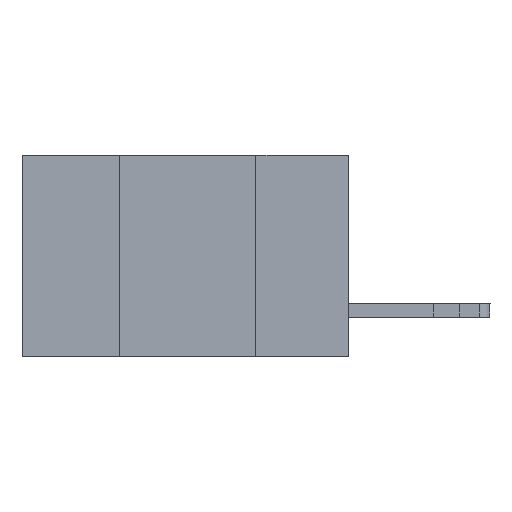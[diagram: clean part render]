
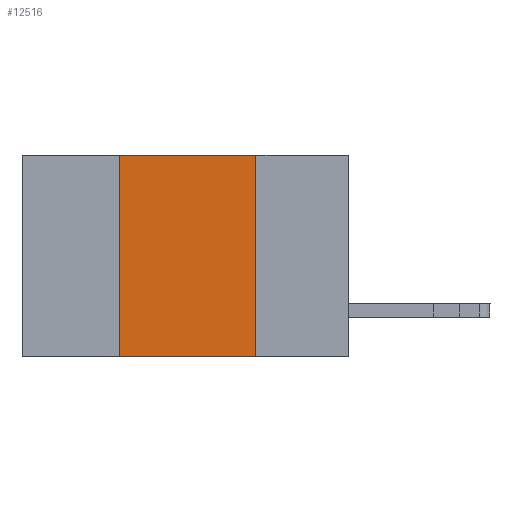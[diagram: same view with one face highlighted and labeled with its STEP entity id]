
A CAD part, left-side view. The second image highlights one B-rep face of the part: STEP entity #12516.
In plain terms, the highlighted planar face has unit normal (-1, 0, 0).
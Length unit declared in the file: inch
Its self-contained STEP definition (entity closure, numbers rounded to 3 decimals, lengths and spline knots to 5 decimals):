
#341 = DIRECTION ( 'NONE',  ( 1., 0., 0. ) ) ;
#452 = CARTESIAN_POINT ( 'NONE',  ( 0., 0.6, 0. ) ) ;
#562 = DIRECTION ( 'NONE',  ( 0., 0., -1. ) ) ;
#1855 = DIRECTION ( 'NONE',  ( 0., 0., 1. ) ) ;
#4172 = VERTEX_POINT ( 'NONE', #7722 ) ;
#4408 = CARTESIAN_POINT ( 'NONE',  ( 0., 0.17, 0. ) ) ;
#4978 = PLANE ( 'NONE',  #6193 ) ;
#5521 = VECTOR ( 'NONE', #16420, 39.37008 ) ;
#5576 = CARTESIAN_POINT ( 'NONE',  ( 0., 0.17, 0. ) ) ;
#6193 = AXIS2_PLACEMENT_3D ( 'NONE', #452, #341, #562 ) ;
#6231 = EDGE_CURVE ( 'NONE', #17138, #4172, #17937, .T. ) ;
#7722 = CARTESIAN_POINT ( 'NONE',  ( 0., 0.42, 0. ) ) ;
#9552 = VECTOR ( 'NONE', #20217, 39.37008 ) ;
#9695 = EDGE_CURVE ( 'NONE', #17138, #19315, #11885, .T. ) ;
#9829 = ORIENTED_EDGE ( 'NONE', *, *, #19598, .F. ) ;
#9984 = LINE ( 'NONE', #11988, #5521 ) ;
#10216 = FACE_OUTER_BOUND ( 'NONE', #20746, .T. ) ;
#11525 = CARTESIAN_POINT ( 'NONE',  ( 0., 0.42, -0.37 ) ) ;
#11875 = VERTEX_POINT ( 'NONE', #4408 ) ;
#11885 = LINE ( 'NONE', #20127, #12164 ) ;
#11988 = CARTESIAN_POINT ( 'NONE',  ( 0., 0.6, 0. ) ) ;
#12164 = VECTOR ( 'NONE', #18324, 39.37008 ) ;
#12516 = ADVANCED_FACE ( 'NONE', ( #10216 ), #4978, .F. ) ;
#12523 = CARTESIAN_POINT ( 'NONE',  ( 0., 0.17, -0.37 ) ) ;
#13143 = EDGE_CURVE ( 'NONE', #11875, #19315, #13459, .T. ) ;
#13459 = LINE ( 'NONE', #5576, #9552 ) ;
#13522 = ORIENTED_EDGE ( 'NONE', *, *, #13143, .F. ) ;
#15099 = ORIENTED_EDGE ( 'NONE', *, *, #9695, .T. ) ;
#15252 = VECTOR ( 'NONE', #1855, 39.37008 ) ;
#15391 = ORIENTED_EDGE ( 'NONE', *, *, #6231, .F. ) ;
#16256 = CARTESIAN_POINT ( 'NONE',  ( 0., 0.42, 0. ) ) ;
#16420 = DIRECTION ( 'NONE',  ( 0., -1., 0. ) ) ;
#17138 = VERTEX_POINT ( 'NONE', #11525 ) ;
#17937 = LINE ( 'NONE', #16256, #15252 ) ;
#18324 = DIRECTION ( 'NONE',  ( 0., -1., 0. ) ) ;
#19315 = VERTEX_POINT ( 'NONE', #12523 ) ;
#19598 = EDGE_CURVE ( 'NONE', #4172, #11875, #9984, .T. ) ;
#20127 = CARTESIAN_POINT ( 'NONE',  ( 0., 0.6, -0.37 ) ) ;
#20217 = DIRECTION ( 'NONE',  ( 0., 0., -1. ) ) ;
#20746 = EDGE_LOOP ( 'NONE', ( #13522, #9829, #15391, #15099 ) ) ;
